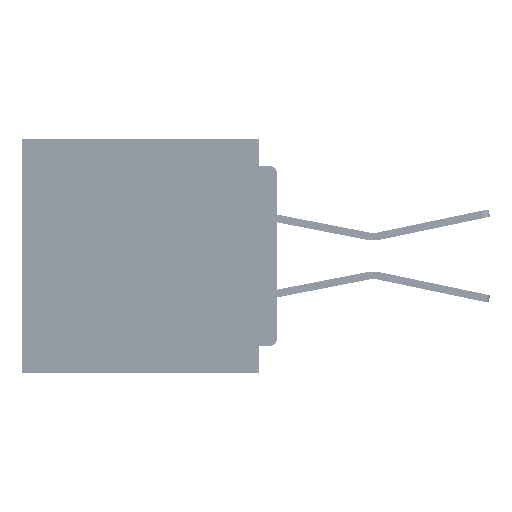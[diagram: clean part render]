
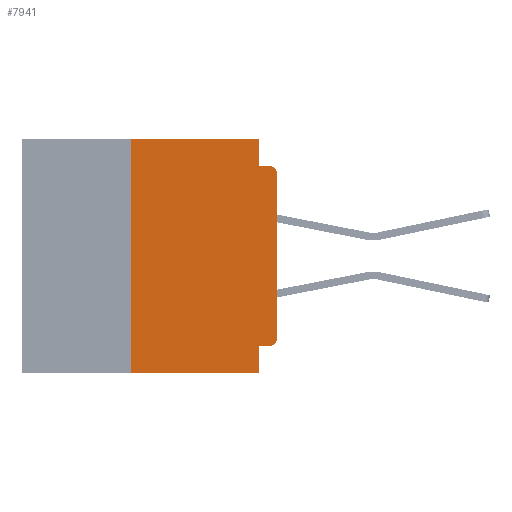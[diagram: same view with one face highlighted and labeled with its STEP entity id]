
A CAD part, left-side view. The second image highlights one B-rep face of the part: STEP entity #7941.
In plain terms, the highlighted planar face has unit normal (-1, 0, 0).
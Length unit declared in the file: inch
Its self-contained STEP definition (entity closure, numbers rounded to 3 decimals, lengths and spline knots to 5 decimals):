
#1652 = ORIENTED_EDGE ( 'NONE', *, *, #35446, .F. ) ;
#2134 = CARTESIAN_POINT ( 'NONE',  ( 0., 0.015, -0.34 ) ) ;
#2365 = EDGE_CURVE ( 'NONE', #29430, #46310, #4626, .T. ) ;
#3144 = CARTESIAN_POINT ( 'NONE',  ( 0., 0.031, -0.045 ) ) ;
#4626 = LINE ( 'NONE', #39160, #30645 ) ;
#4822 = EDGE_CURVE ( 'NONE', #52570, #6734, #4948, .T. ) ;
#4948 = LINE ( 'NONE', #16646, #60118 ) ;
#6561 = VERTEX_POINT ( 'NONE', #43193 ) ;
#6734 = VERTEX_POINT ( 'NONE', #3144 ) ;
#7470 = DIRECTION ( 'NONE',  ( 0., 0., -1. ) ) ;
#7512 = CARTESIAN_POINT ( 'NONE',  ( 0., 0.25, -0.4 ) ) ;
#7751 = VECTOR ( 'NONE', #58314, 39.37008 ) ;
#7941 = ADVANCED_FACE ( 'NONE', ( #16538 ), #44136, .F. ) ;
#8039 = LINE ( 'NONE', #61556, #61514 ) ;
#9379 = LINE ( 'NONE', #17103, #7751 ) ;
#10318 = CARTESIAN_POINT ( 'NONE',  ( 0., 0.031, -0.4 ) ) ;
#10523 = CARTESIAN_POINT ( 'NONE',  ( 0., 0., 0. ) ) ;
#11395 = CARTESIAN_POINT ( 'NONE',  ( 0., 0.25, 0. ) ) ;
#11592 = DIRECTION ( 'NONE',  ( -1., 0., 0. ) ) ;
#12237 = DIRECTION ( 'NONE',  ( 0., -1., 0. ) ) ;
#12436 = ORIENTED_EDGE ( 'NONE', *, *, #38263, .T. ) ;
#12512 = EDGE_CURVE ( 'NONE', #16673, #48918, #9379, .T. ) ;
#13092 = DIRECTION ( 'NONE',  ( 1., 0., 0. ) ) ;
#14041 = CIRCLE ( 'NONE', #31389, 0.015 ) ;
#14147 = EDGE_CURVE ( 'NONE', #48918, #62048, #43425, .T. ) ;
#15446 = VERTEX_POINT ( 'NONE', #42313 ) ;
#16538 = FACE_OUTER_BOUND ( 'NONE', #21413, .T. ) ;
#16646 = CARTESIAN_POINT ( 'NONE',  ( 0., 0.031, 0. ) ) ;
#16673 = VERTEX_POINT ( 'NONE', #62235 ) ;
#17103 = CARTESIAN_POINT ( 'NONE',  ( 0., 0., -0.355 ) ) ;
#17858 = CARTESIAN_POINT ( 'NONE',  ( 0., 0.437, 0. ) ) ;
#21413 = EDGE_LOOP ( 'NONE', ( #43698, #64326, #1652, #36431, #49649, #66456, #12436, #39507, #38416, #43413 ) ) ;
#22399 = VERTEX_POINT ( 'NONE', #42357 ) ;
#28945 = VECTOR ( 'NONE', #12237, 39.37008 ) ;
#29062 = VECTOR ( 'NONE', #51981, 39.37008 ) ;
#29430 = VERTEX_POINT ( 'NONE', #7512 ) ;
#29632 = VECTOR ( 'NONE', #46584, 39.37008 ) ;
#30645 = VECTOR ( 'NONE', #54770, 39.37008 ) ;
#31389 = AXIS2_PLACEMENT_3D ( 'NONE', #2134, #38555, #7470 ) ;
#31515 = AXIS2_PLACEMENT_3D ( 'NONE', #42667, #11592, #47848 ) ;
#32068 = CARTESIAN_POINT ( 'NONE',  ( 0., 0.031, 0. ) ) ;
#32854 = DIRECTION ( 'NONE',  ( 0., -1., 0. ) ) ;
#33291 = EDGE_CURVE ( 'NONE', #16673, #22399, #14041, .T. ) ;
#34425 = CARTESIAN_POINT ( 'NONE',  ( 0., 0.031, -0.355 ) ) ;
#34977 = EDGE_CURVE ( 'NONE', #6561, #15446, #47845, .T. ) ;
#35446 = EDGE_CURVE ( 'NONE', #6734, #15446, #8039, .T. ) ;
#36431 = ORIENTED_EDGE ( 'NONE', *, *, #4822, .F. ) ;
#38263 = EDGE_CURVE ( 'NONE', #29430, #62048, #40222, .T. ) ;
#38416 = ORIENTED_EDGE ( 'NONE', *, *, #12512, .F. ) ;
#38555 = DIRECTION ( 'NONE',  ( -1., 0., 0. ) ) ;
#39160 = CARTESIAN_POINT ( 'NONE',  ( 0., 0.25, -0.4 ) ) ;
#39507 = ORIENTED_EDGE ( 'NONE', *, *, #14147, .F. ) ;
#40222 = LINE ( 'NONE', #58635, #66033 ) ;
#41400 = AXIS2_PLACEMENT_3D ( 'NONE', #17858, #13092, #49317 ) ;
#42313 = CARTESIAN_POINT ( 'NONE',  ( 0., 0.015, -0.045 ) ) ;
#42357 = CARTESIAN_POINT ( 'NONE',  ( 0., 0., -0.34 ) ) ;
#42667 = CARTESIAN_POINT ( 'NONE',  ( 0., 0.015, -0.06 ) ) ;
#43193 = CARTESIAN_POINT ( 'NONE',  ( 0., 0., -0.06 ) ) ;
#43413 = ORIENTED_EDGE ( 'NONE', *, *, #33291, .T. ) ;
#43425 = LINE ( 'NONE', #10318, #29632 ) ;
#43698 = ORIENTED_EDGE ( 'NONE', *, *, #50718, .T. ) ;
#44136 = PLANE ( 'NONE',  #41400 ) ;
#44473 = LINE ( 'NONE', #10523, #29062 ) ;
#46310 = VERTEX_POINT ( 'NONE', #11395 ) ;
#46584 = DIRECTION ( 'NONE',  ( 0., 0., -1. ) ) ;
#47845 = CIRCLE ( 'NONE', #31515, 0.015 ) ;
#47848 = DIRECTION ( 'NONE',  ( 0., 0., -1. ) ) ;
#48918 = VERTEX_POINT ( 'NONE', #34425 ) ;
#49317 = DIRECTION ( 'NONE',  ( 0., 0., -1. ) ) ;
#49649 = ORIENTED_EDGE ( 'NONE', *, *, #51526, .F. ) ;
#50718 = EDGE_CURVE ( 'NONE', #22399, #6561, #44473, .T. ) ;
#51388 = CARTESIAN_POINT ( 'NONE',  ( 0., 0.031, -0.4 ) ) ;
#51526 = EDGE_CURVE ( 'NONE', #46310, #52570, #56508, .T. ) ;
#51981 = DIRECTION ( 'NONE',  ( 0., 0., 1. ) ) ;
#52570 = VERTEX_POINT ( 'NONE', #32068 ) ;
#52874 = DIRECTION ( 'NONE',  ( 0., 0., -1. ) ) ;
#54770 = DIRECTION ( 'NONE',  ( 0., 0., 1. ) ) ;
#56508 = LINE ( 'NONE', #64034, #28945 ) ;
#56637 = DIRECTION ( 'NONE',  ( 0., -1., 0. ) ) ;
#58314 = DIRECTION ( 'NONE',  ( 0., 1., 0. ) ) ;
#58635 = CARTESIAN_POINT ( 'NONE',  ( 0., 0.437, -0.4 ) ) ;
#60118 = VECTOR ( 'NONE', #52874, 39.37008 ) ;
#61514 = VECTOR ( 'NONE', #56637, 39.37008 ) ;
#61556 = CARTESIAN_POINT ( 'NONE',  ( 0., 0., -0.045 ) ) ;
#62048 = VERTEX_POINT ( 'NONE', #51388 ) ;
#62235 = CARTESIAN_POINT ( 'NONE',  ( 0., 0.015, -0.355 ) ) ;
#64034 = CARTESIAN_POINT ( 'NONE',  ( 0., 0.437, 0. ) ) ;
#64326 = ORIENTED_EDGE ( 'NONE', *, *, #34977, .T. ) ;
#66033 = VECTOR ( 'NONE', #32854, 39.37008 ) ;
#66456 = ORIENTED_EDGE ( 'NONE', *, *, #2365, .F. ) ;
